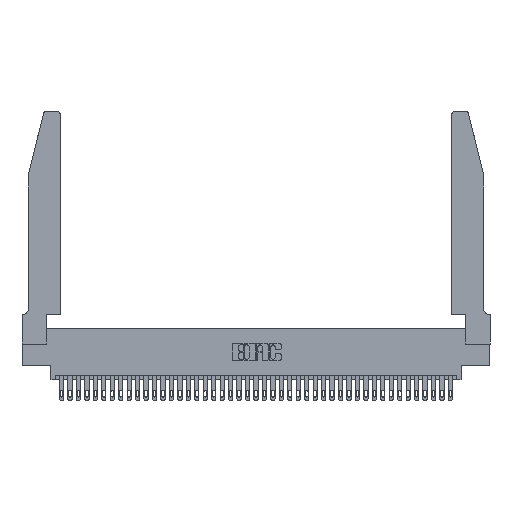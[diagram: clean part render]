
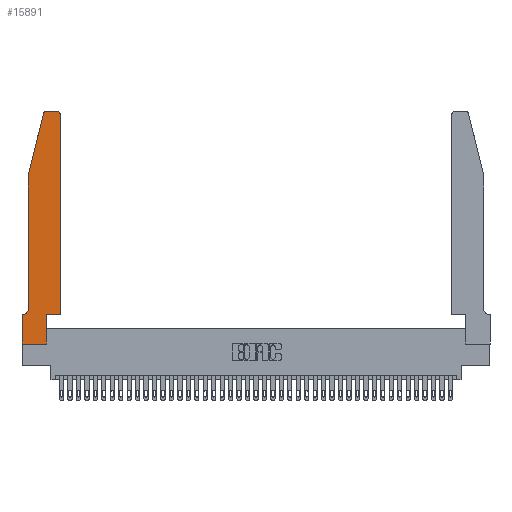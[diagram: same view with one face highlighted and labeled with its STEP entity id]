
A CAD part, top view. The second image highlights one B-rep face of the part: STEP entity #15891.
In plain terms, the highlighted planar face has unit normal (0, 0, 1).
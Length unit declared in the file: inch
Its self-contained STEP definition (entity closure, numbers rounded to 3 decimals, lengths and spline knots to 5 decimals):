
#3 = EDGE_CURVE ( 'NONE', #10634, #29055, #2147, .T. ) ;
#362 = AXIS2_PLACEMENT_3D ( 'NONE', #14172, #29726, #33333 ) ;
#1122 = VERTEX_POINT ( 'NONE', #2350 ) ;
#1250 = DIRECTION ( 'NONE',  ( 0., 0., 1. ) ) ;
#1552 = VECTOR ( 'NONE', #11589, 39.37008 ) ;
#1994 = EDGE_LOOP ( 'NONE', ( #12531, #34467, #30032, #19073, #7927, #8300, #11508, #15939, #34332, #30756, #16281, #19241 ) ) ;
#2035 = DIRECTION ( 'NONE',  ( 0., 0., -1. ) ) ;
#2139 = CARTESIAN_POINT ( 'NONE',  ( 0.4505, 0.35, 0.37 ) ) ;
#2147 = CIRCLE ( 'NONE', #29719, 0.07 ) ;
#2350 = CARTESIAN_POINT ( 'NONE',  ( 0.0755, 2., 0.37 ) ) ;
#2851 = EDGE_CURVE ( 'NONE', #13959, #17611, #10755, .T. ) ;
#3050 = EDGE_CURVE ( 'NONE', #30638, #30421, #16644, .T. ) ;
#4983 = CARTESIAN_POINT ( 'NONE',  ( 0.284, 2.72, 0.37 ) ) ;
#5115 = VERTEX_POINT ( 'NONE', #21847 ) ;
#5689 = VERTEX_POINT ( 'NONE', #36513 ) ;
#5913 = DIRECTION ( 'NONE',  ( 0., -1., 0. ) ) ;
#6706 = CIRCLE ( 'NONE', #13509, 0.03 ) ;
#7927 = ORIENTED_EDGE ( 'NONE', *, *, #3, .T. ) ;
#8227 = CARTESIAN_POINT ( 'NONE',  ( 0.4205, 2.72, 0.37 ) ) ;
#8300 = ORIENTED_EDGE ( 'NONE', *, *, #28222, .T. ) ;
#8828 = CARTESIAN_POINT ( 'NONE',  ( 0.4505, 0.35, 0.37 ) ) ;
#10634 = VERTEX_POINT ( 'NONE', #14488 ) ;
#10635 = DIRECTION ( 'NONE',  ( 1., 0., 0. ) ) ;
#10755 = LINE ( 'NONE', #12230, #20120 ) ;
#10939 = CARTESIAN_POINT ( 'NONE',  ( 0.4505, 2.72, 0.37 ) ) ;
#11439 = EDGE_CURVE ( 'NONE', #15967, #5689, #6706, .T. ) ;
#11508 = ORIENTED_EDGE ( 'NONE', *, *, #24271, .T. ) ;
#11525 = DIRECTION ( 'NONE',  ( -1., 0., 0. ) ) ;
#11589 = DIRECTION ( 'NONE',  ( 1., 0., 0. ) ) ;
#12101 = CIRCLE ( 'NONE', #29348, 0.03 ) ;
#12230 = CARTESIAN_POINT ( 'NONE',  ( 0.2865, 0.35, 0.37 ) ) ;
#12424 = DIRECTION ( 'NONE',  ( 1., 0., 0. ) ) ;
#12508 = VECTOR ( 'NONE', #41042, 39.37008 ) ;
#12531 = ORIENTED_EDGE ( 'NONE', *, *, #29949, .T. ) ;
#13509 = AXIS2_PLACEMENT_3D ( 'NONE', #4983, #1250, #10635 ) ;
#13612 = LINE ( 'NONE', #31150, #25993 ) ;
#13959 = VERTEX_POINT ( 'NONE', #31615 ) ;
#14172 = CARTESIAN_POINT ( 'NONE',  ( 0., 0.35, 0.37 ) ) ;
#14488 = CARTESIAN_POINT ( 'NONE',  ( 0.0755, 0.42, 0.37 ) ) ;
#15800 = DIRECTION ( 'NONE',  ( -1., 0., 0. ) ) ;
#15889 = LINE ( 'NONE', #8828, #1552 ) ;
#15891 = ADVANCED_FACE ( 'NONE', ( #24596 ), #33061, .T. ) ;
#15939 = ORIENTED_EDGE ( 'NONE', *, *, #27438, .T. ) ;
#15967 = VERTEX_POINT ( 'NONE', #20927 ) ;
#16281 = ORIENTED_EDGE ( 'NONE', *, *, #3050, .T. ) ;
#16421 = CARTESIAN_POINT ( 'NONE',  ( 0., 0.35, 0.37 ) ) ;
#16644 = LINE ( 'NONE', #2139, #32588 ) ;
#17611 = VERTEX_POINT ( 'NONE', #28607 ) ;
#17839 = CARTESIAN_POINT ( 'NONE',  ( 0.4505, 0.35, 0.37 ) ) ;
#18119 = LINE ( 'NONE', #32436, #28569 ) ;
#18560 = EDGE_CURVE ( 'NONE', #5689, #1122, #24922, .T. ) ;
#19073 = ORIENTED_EDGE ( 'NONE', *, *, #34560, .T. ) ;
#19241 = ORIENTED_EDGE ( 'NONE', *, *, #29814, .T. ) ;
#20120 = VECTOR ( 'NONE', #34597, 39.37008 ) ;
#20927 = CARTESIAN_POINT ( 'NONE',  ( 0.284, 2.75, 0.37 ) ) ;
#21101 = EDGE_CURVE ( 'NONE', #17611, #30638, #15889, .T. ) ;
#21806 = CARTESIAN_POINT ( 'NONE',  ( 0., 0., 0.37 ) ) ;
#21847 = CARTESIAN_POINT ( 'NONE',  ( 0.4205, 2.75, 0.37 ) ) ;
#22756 = VERTEX_POINT ( 'NONE', #25667 ) ;
#23565 = DIRECTION ( 'NONE',  ( 0., 0., 1. ) ) ;
#24109 = LINE ( 'NONE', #40961, #25109 ) ;
#24271 = EDGE_CURVE ( 'NONE', #34568, #22756, #13612, .T. ) ;
#24596 = FACE_OUTER_BOUND ( 'NONE', #1994, .T. ) ;
#24922 = LINE ( 'NONE', #27844, #12508 ) ;
#25109 = VECTOR ( 'NONE', #15800, 39.37008 ) ;
#25667 = CARTESIAN_POINT ( 'NONE',  ( 0., 0., 0.37 ) ) ;
#25993 = VECTOR ( 'NONE', #5913, 39.37008 ) ;
#27149 = VECTOR ( 'NONE', #12424, 39.37008 ) ;
#27438 = EDGE_CURVE ( 'NONE', #22756, #13959, #35628, .T. ) ;
#27844 = CARTESIAN_POINT ( 'NONE',  ( 0.0755, 2., 0.37 ) ) ;
#27886 = CARTESIAN_POINT ( 'NONE',  ( 0.2605, 2.75, 0.37 ) ) ;
#28222 = EDGE_CURVE ( 'NONE', #29055, #34568, #24109, .T. ) ;
#28452 = LINE ( 'NONE', #27886, #31469 ) ;
#28569 = VECTOR ( 'NONE', #32297, 39.37008 ) ;
#28607 = CARTESIAN_POINT ( 'NONE',  ( 0.2865, 0.35, 0.37 ) ) ;
#29055 = VERTEX_POINT ( 'NONE', #38499 ) ;
#29348 = AXIS2_PLACEMENT_3D ( 'NONE', #8227, #23565, #29972 ) ;
#29719 = AXIS2_PLACEMENT_3D ( 'NONE', #33598, #2035, #11525 ) ;
#29726 = DIRECTION ( 'NONE',  ( 0., 0., 1. ) ) ;
#29814 = EDGE_CURVE ( 'NONE', #30421, #5115, #12101, .T. ) ;
#29949 = EDGE_CURVE ( 'NONE', #5115, #15967, #28452, .T. ) ;
#29972 = DIRECTION ( 'NONE',  ( 1., 0., 0. ) ) ;
#30032 = ORIENTED_EDGE ( 'NONE', *, *, #18560, .T. ) ;
#30421 = VERTEX_POINT ( 'NONE', #10939 ) ;
#30638 = VERTEX_POINT ( 'NONE', #17839 ) ;
#30756 = ORIENTED_EDGE ( 'NONE', *, *, #21101, .T. ) ;
#31150 = CARTESIAN_POINT ( 'NONE',  ( 0., 0., 0.37 ) ) ;
#31469 = VECTOR ( 'NONE', #37516, 39.37008 ) ;
#31615 = CARTESIAN_POINT ( 'NONE',  ( 0.2865, 0., 0.37 ) ) ;
#32297 = DIRECTION ( 'NONE',  ( 0., -1., 0. ) ) ;
#32436 = CARTESIAN_POINT ( 'NONE',  ( 0.0755, 2., 0.37 ) ) ;
#32588 = VECTOR ( 'NONE', #40361, 39.37008 ) ;
#33061 = PLANE ( 'NONE',  #362 ) ;
#33333 = DIRECTION ( 'NONE',  ( 1., 0., 0. ) ) ;
#33598 = CARTESIAN_POINT ( 'NONE',  ( 0.0055, 0.42, 0.37 ) ) ;
#34332 = ORIENTED_EDGE ( 'NONE', *, *, #2851, .T. ) ;
#34467 = ORIENTED_EDGE ( 'NONE', *, *, #11439, .T. ) ;
#34560 = EDGE_CURVE ( 'NONE', #1122, #10634, #18119, .T. ) ;
#34568 = VERTEX_POINT ( 'NONE', #16421 ) ;
#34597 = DIRECTION ( 'NONE',  ( 0., 1., 0. ) ) ;
#35628 = LINE ( 'NONE', #21806, #27149 ) ;
#36513 = CARTESIAN_POINT ( 'NONE',  ( 0.25487, 2.72718, 0.37 ) ) ;
#37516 = DIRECTION ( 'NONE',  ( -1., 0., 0. ) ) ;
#38499 = CARTESIAN_POINT ( 'NONE',  ( 0.0055, 0.35, 0.37 ) ) ;
#40361 = DIRECTION ( 'NONE',  ( 0., 1., 0. ) ) ;
#40961 = CARTESIAN_POINT ( 'NONE',  ( 0.0755, 0.35, 0.37 ) ) ;
#41042 = DIRECTION ( 'NONE',  ( -0.239, -0.971, 0. ) ) ;
